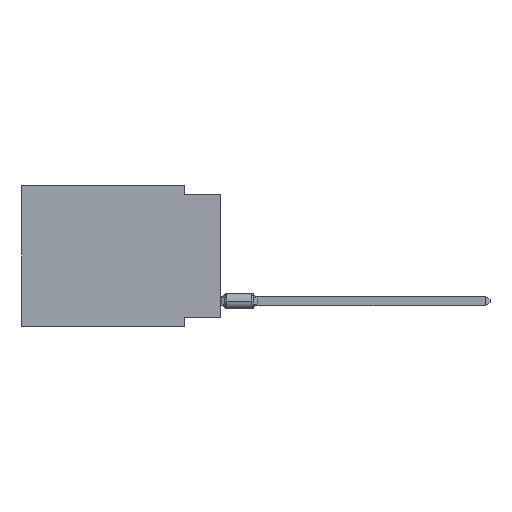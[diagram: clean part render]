
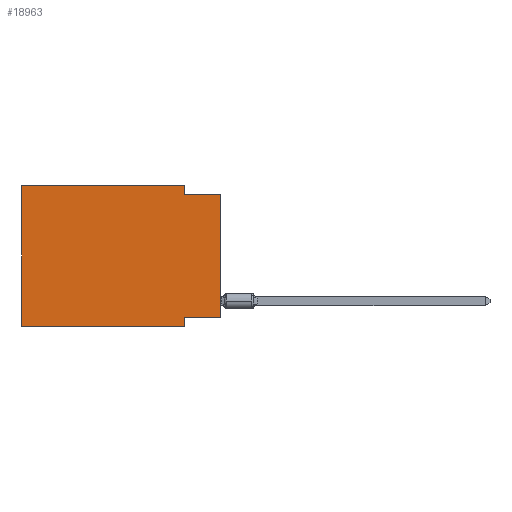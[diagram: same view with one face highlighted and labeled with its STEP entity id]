
A CAD part, left-side view. The second image highlights one B-rep face of the part: STEP entity #18963.
In plain terms, the highlighted planar face has unit normal (-1, 0, 0).
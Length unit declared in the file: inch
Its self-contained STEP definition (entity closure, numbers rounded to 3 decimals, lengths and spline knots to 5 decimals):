
#51 = CARTESIAN_POINT ( 'NONE',  ( 0., 0.1, -0.39 ) ) ;
#367 = AXIS2_PLACEMENT_3D ( 'NONE', #16664, #30882, #30715 ) ;
#1435 = CARTESIAN_POINT ( 'NONE',  ( 0., 0.1, -0.025 ) ) ;
#1889 = EDGE_CURVE ( 'NONE', #26598, #21307, #18930, .T. ) ;
#2844 = EDGE_CURVE ( 'NONE', #11100, #33774, #31972, .T. ) ;
#3081 = DIRECTION ( 'NONE',  ( 0., 0., 1. ) ) ;
#3924 = VERTEX_POINT ( 'NONE', #18153 ) ;
#4277 = ORIENTED_EDGE ( 'NONE', *, *, #29320, .F. ) ;
#4758 = ORIENTED_EDGE ( 'NONE', *, *, #25701, .F. ) ;
#4867 = CARTESIAN_POINT ( 'NONE',  ( 0., 0.1, -0.39 ) ) ;
#6694 = VERTEX_POINT ( 'NONE', #12632 ) ;
#7144 = VERTEX_POINT ( 'NONE', #29023 ) ;
#7430 = LINE ( 'NONE', #21482, #32583 ) ;
#7444 = LINE ( 'NONE', #28982, #32663 ) ;
#8031 = ORIENTED_EDGE ( 'NONE', *, *, #2844, .T. ) ;
#8509 = CARTESIAN_POINT ( 'NONE',  ( 0., 0., -0.025 ) ) ;
#9913 = EDGE_CURVE ( 'NONE', #3924, #27977, #21495, .T. ) ;
#9981 = DIRECTION ( 'NONE',  ( 0., -1., 0. ) ) ;
#10386 = EDGE_LOOP ( 'NONE', ( #8031, #16378, #26440, #4758, #4277, #33583, #33445, #17890 ) ) ;
#11100 = VERTEX_POINT ( 'NONE', #24399 ) ;
#12632 = CARTESIAN_POINT ( 'NONE',  ( 0., 0.55, 0. ) ) ;
#12795 = EDGE_CURVE ( 'NONE', #7144, #21307, #33668, .T. ) ;
#14069 = CARTESIAN_POINT ( 'NONE',  ( 0., 0.1, -0.365 ) ) ;
#15459 = DIRECTION ( 'NONE',  ( 0., 1., 0. ) ) ;
#15532 = DIRECTION ( 'NONE',  ( 0., -1., 0. ) ) ;
#16378 = ORIENTED_EDGE ( 'NONE', *, *, #35432, .F. ) ;
#16664 = CARTESIAN_POINT ( 'NONE',  ( 0., 0.55, 0. ) ) ;
#17890 = ORIENTED_EDGE ( 'NONE', *, *, #22342, .F. ) ;
#18153 = CARTESIAN_POINT ( 'NONE',  ( 0., 0.1, 0. ) ) ;
#18404 = VECTOR ( 'NONE', #33306, 39.37008 ) ;
#18930 = LINE ( 'NONE', #4867, #21311 ) ;
#18963 = ADVANCED_FACE ( 'NONE', ( #19774 ), #25571, .F. ) ;
#19074 = CARTESIAN_POINT ( 'NONE',  ( 0., 0., -0.025 ) ) ;
#19531 = CARTESIAN_POINT ( 'NONE',  ( 0., 0.55, 0. ) ) ;
#19774 = FACE_OUTER_BOUND ( 'NONE', #10386, .T. ) ;
#21046 = VECTOR ( 'NONE', #27143, 39.37008 ) ;
#21307 = VERTEX_POINT ( 'NONE', #51 ) ;
#21311 = VECTOR ( 'NONE', #32409, 39.37008 ) ;
#21482 = CARTESIAN_POINT ( 'NONE',  ( 0., 0., -0.365 ) ) ;
#21495 = LINE ( 'NONE', #32604, #21046 ) ;
#22342 = EDGE_CURVE ( 'NONE', #11100, #26598, #7430, .T. ) ;
#22879 = VECTOR ( 'NONE', #15532, 39.37008 ) ;
#24399 = CARTESIAN_POINT ( 'NONE',  ( 0., 0., -0.365 ) ) ;
#24611 = VECTOR ( 'NONE', #3081, 39.37008 ) ;
#25163 = LINE ( 'NONE', #19531, #24611 ) ;
#25571 = PLANE ( 'NONE',  #367 ) ;
#25701 = EDGE_CURVE ( 'NONE', #6694, #3924, #7444, .T. ) ;
#25937 = CARTESIAN_POINT ( 'NONE',  ( 0., 0.55, -0.39 ) ) ;
#26440 = ORIENTED_EDGE ( 'NONE', *, *, #9913, .F. ) ;
#26598 = VERTEX_POINT ( 'NONE', #14069 ) ;
#27143 = DIRECTION ( 'NONE',  ( 0., 0., -1. ) ) ;
#27977 = VERTEX_POINT ( 'NONE', #1435 ) ;
#28982 = CARTESIAN_POINT ( 'NONE',  ( 0., 0.55, 0. ) ) ;
#29023 = CARTESIAN_POINT ( 'NONE',  ( 0., 0.55, -0.39 ) ) ;
#29320 = EDGE_CURVE ( 'NONE', #7144, #6694, #25163, .T. ) ;
#30715 = DIRECTION ( 'NONE',  ( 0., 0., -1. ) ) ;
#30882 = DIRECTION ( 'NONE',  ( 1., 0., 0. ) ) ;
#31793 = CARTESIAN_POINT ( 'NONE',  ( 0., 0., 0. ) ) ;
#31972 = LINE ( 'NONE', #31793, #32548 ) ;
#32328 = DIRECTION ( 'NONE',  ( 0., 0., 1. ) ) ;
#32409 = DIRECTION ( 'NONE',  ( 0., 0., -1. ) ) ;
#32548 = VECTOR ( 'NONE', #32328, 39.37008 ) ;
#32583 = VECTOR ( 'NONE', #15459, 39.37008 ) ;
#32604 = CARTESIAN_POINT ( 'NONE',  ( 0., 0.1, 0. ) ) ;
#32663 = VECTOR ( 'NONE', #9981, 39.37008 ) ;
#33306 = DIRECTION ( 'NONE',  ( 0., -1., 0. ) ) ;
#33445 = ORIENTED_EDGE ( 'NONE', *, *, #1889, .F. ) ;
#33496 = LINE ( 'NONE', #8509, #18404 ) ;
#33583 = ORIENTED_EDGE ( 'NONE', *, *, #12795, .T. ) ;
#33668 = LINE ( 'NONE', #25937, #22879 ) ;
#33774 = VERTEX_POINT ( 'NONE', #19074 ) ;
#35432 = EDGE_CURVE ( 'NONE', #27977, #33774, #33496, .T. ) ;
